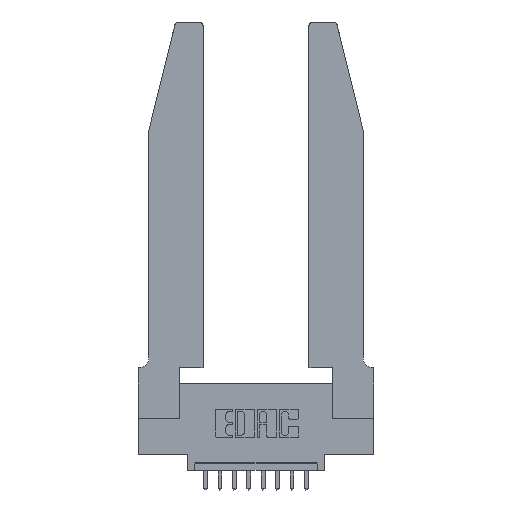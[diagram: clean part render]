
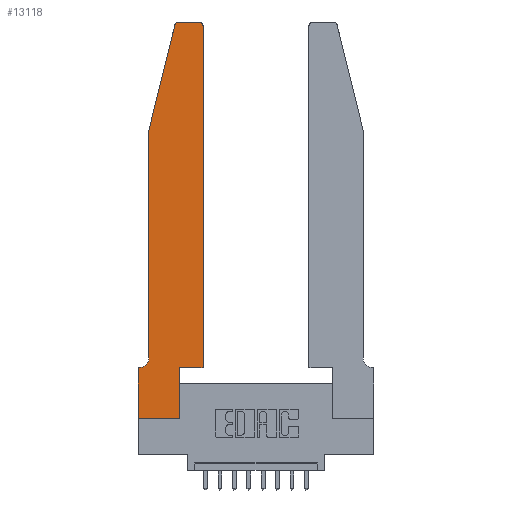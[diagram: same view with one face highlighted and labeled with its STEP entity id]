
A CAD part, top view. The second image highlights one B-rep face of the part: STEP entity #13118.
In plain terms, the highlighted planar face has unit normal (0, 0, 1).
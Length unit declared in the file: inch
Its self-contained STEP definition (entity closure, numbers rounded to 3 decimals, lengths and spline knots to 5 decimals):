
#37 = CARTESIAN_POINT ( 'NONE',  ( 0.0055, 0.42, 0.37 ) ) ;
#318 = ORIENTED_EDGE ( 'NONE', *, *, #5589, .T. ) ;
#415 = VECTOR ( 'NONE', #8741, 39.37008 ) ;
#494 = ORIENTED_EDGE ( 'NONE', *, *, #6940, .T. ) ;
#845 = ORIENTED_EDGE ( 'NONE', *, *, #9749, .T. ) ;
#1042 = DIRECTION ( 'NONE',  ( 0., 0., 1. ) ) ;
#1146 = CARTESIAN_POINT ( 'NONE',  ( 0.284, 2.72, 0.37 ) ) ;
#1569 = PLANE ( 'NONE',  #14607 ) ;
#1967 = VERTEX_POINT ( 'NONE', #10057 ) ;
#1981 = CIRCLE ( 'NONE', #5795, 0.07 ) ;
#2119 = VERTEX_POINT ( 'NONE', #8149 ) ;
#2157 = EDGE_CURVE ( 'NONE', #10383, #11091, #13105, .T. ) ;
#2395 = ORIENTED_EDGE ( 'NONE', *, *, #12635, .T. ) ;
#2625 = VECTOR ( 'NONE', #10689, 39.37008 ) ;
#2640 = VERTEX_POINT ( 'NONE', #8347 ) ;
#2747 = VERTEX_POINT ( 'NONE', #4950 ) ;
#2975 = FACE_OUTER_BOUND ( 'NONE', #6156, .T. ) ;
#3024 = CARTESIAN_POINT ( 'NONE',  ( 0.4505, 2.72, 0.37 ) ) ;
#3044 = AXIS2_PLACEMENT_3D ( 'NONE', #1146, #1042, #4704 ) ;
#3399 = EDGE_CURVE ( 'NONE', #11091, #9227, #14412, .T. ) ;
#3501 = DIRECTION ( 'NONE',  ( -0.239, -0.971, 0. ) ) ;
#3554 = VECTOR ( 'NONE', #3501, 39.37008 ) ;
#3577 = LINE ( 'NONE', #6527, #7161 ) ;
#3654 = DIRECTION ( 'NONE',  ( 0., 1., 0. ) ) ;
#3967 = CARTESIAN_POINT ( 'NONE',  ( 0., 0.35, 0.37 ) ) ;
#4281 = EDGE_CURVE ( 'NONE', #1967, #6999, #15196, .T. ) ;
#4324 = VECTOR ( 'NONE', #12810, 39.37008 ) ;
#4589 = ORIENTED_EDGE ( 'NONE', *, *, #2157, .T. ) ;
#4704 = DIRECTION ( 'NONE',  ( 1., 0., 0. ) ) ;
#4751 = DIRECTION ( 'NONE',  ( -1., 0., 0. ) ) ;
#4950 = CARTESIAN_POINT ( 'NONE',  ( 0.0755, 2., 0.37 ) ) ;
#4961 = ORIENTED_EDGE ( 'NONE', *, *, #12602, .T. ) ;
#5038 = CARTESIAN_POINT ( 'NONE',  ( 0.2865, 0.35, 0.37 ) ) ;
#5060 = DIRECTION ( 'NONE',  ( 0., 1., 0. ) ) ;
#5204 = DIRECTION ( 'NONE',  ( 0., 0., 1. ) ) ;
#5482 = CARTESIAN_POINT ( 'NONE',  ( 0.284, 2.75, 0.37 ) ) ;
#5589 = EDGE_CURVE ( 'NONE', #2747, #2640, #9210, .T. ) ;
#5600 = ORIENTED_EDGE ( 'NONE', *, *, #12758, .T. ) ;
#5795 = AXIS2_PLACEMENT_3D ( 'NONE', #37, #8422, #10828 ) ;
#6007 = LINE ( 'NONE', #9488, #2625 ) ;
#6156 = EDGE_LOOP ( 'NONE', ( #14097, #5600, #4961, #318, #7745, #8527, #8144, #2395, #845, #494, #11410, #4589 ) ) ;
#6436 = DIRECTION ( 'NONE',  ( 0., -1., 0. ) ) ;
#6527 = CARTESIAN_POINT ( 'NONE',  ( 0., 0., 0.37 ) ) ;
#6940 = EDGE_CURVE ( 'NONE', #12651, #11143, #6007, .T. ) ;
#6999 = VERTEX_POINT ( 'NONE', #10043 ) ;
#7033 = CARTESIAN_POINT ( 'NONE',  ( 0.25487, 2.72718, 0.37 ) ) ;
#7161 = VECTOR ( 'NONE', #6436, 39.37008 ) ;
#7534 = VECTOR ( 'NONE', #3654, 39.37008 ) ;
#7745 = ORIENTED_EDGE ( 'NONE', *, *, #15525, .T. ) ;
#8099 = CARTESIAN_POINT ( 'NONE',  ( 0.4205, 2.72, 0.37 ) ) ;
#8144 = ORIENTED_EDGE ( 'NONE', *, *, #11043, .T. ) ;
#8149 = CARTESIAN_POINT ( 'NONE',  ( 0.2865, 0., 0.37 ) ) ;
#8242 = AXIS2_PLACEMENT_3D ( 'NONE', #8099, #12911, #14119 ) ;
#8347 = CARTESIAN_POINT ( 'NONE',  ( 0.0755, 0.42, 0.37 ) ) ;
#8422 = DIRECTION ( 'NONE',  ( 0., 0., -1. ) ) ;
#8527 = ORIENTED_EDGE ( 'NONE', *, *, #4281, .T. ) ;
#8741 = DIRECTION ( 'NONE',  ( -1., 0., 0. ) ) ;
#8923 = VERTEX_POINT ( 'NONE', #7033 ) ;
#8940 = CARTESIAN_POINT ( 'NONE',  ( 0.0755, 0.35, 0.37 ) ) ;
#8990 = VECTOR ( 'NONE', #9888, 39.37008 ) ;
#9210 = LINE ( 'NONE', #10341, #4324 ) ;
#9227 = VERTEX_POINT ( 'NONE', #5482 ) ;
#9481 = CARTESIAN_POINT ( 'NONE',  ( 0.0755, 2., 0.37 ) ) ;
#9488 = CARTESIAN_POINT ( 'NONE',  ( 0.4505, 0.35, 0.37 ) ) ;
#9523 = CARTESIAN_POINT ( 'NONE',  ( 0.2605, 2.75, 0.37 ) ) ;
#9749 = EDGE_CURVE ( 'NONE', #2119, #12651, #11343, .T. ) ;
#9888 = DIRECTION ( 'NONE',  ( 1., 0., 0. ) ) ;
#10043 = CARTESIAN_POINT ( 'NONE',  ( 0., 0.35, 0.37 ) ) ;
#10057 = CARTESIAN_POINT ( 'NONE',  ( 0.0055, 0.35, 0.37 ) ) ;
#10307 = LINE ( 'NONE', #9481, #3554 ) ;
#10341 = CARTESIAN_POINT ( 'NONE',  ( 0.0755, 2., 0.37 ) ) ;
#10383 = VERTEX_POINT ( 'NONE', #3024 ) ;
#10608 = CARTESIAN_POINT ( 'NONE',  ( 0.4505, 0.35, 0.37 ) ) ;
#10689 = DIRECTION ( 'NONE',  ( 1., 0., 0. ) ) ;
#10692 = LINE ( 'NONE', #10838, #7534 ) ;
#10828 = DIRECTION ( 'NONE',  ( -1., 0., 0. ) ) ;
#10838 = CARTESIAN_POINT ( 'NONE',  ( 0.4505, 0.35, 0.37 ) ) ;
#10893 = CARTESIAN_POINT ( 'NONE',  ( 0., 0., 0.37 ) ) ;
#11043 = EDGE_CURVE ( 'NONE', #6999, #12601, #3577, .T. ) ;
#11087 = LINE ( 'NONE', #10893, #8990 ) ;
#11091 = VERTEX_POINT ( 'NONE', #13747 ) ;
#11143 = VERTEX_POINT ( 'NONE', #10608 ) ;
#11153 = VECTOR ( 'NONE', #5060, 39.37008 ) ;
#11252 = CIRCLE ( 'NONE', #3044, 0.03 ) ;
#11343 = LINE ( 'NONE', #13457, #11153 ) ;
#11410 = ORIENTED_EDGE ( 'NONE', *, *, #12582, .T. ) ;
#11848 = CARTESIAN_POINT ( 'NONE',  ( 0., 0., 0.37 ) ) ;
#12582 = EDGE_CURVE ( 'NONE', #11143, #10383, #10692, .T. ) ;
#12601 = VERTEX_POINT ( 'NONE', #11848 ) ;
#12602 = EDGE_CURVE ( 'NONE', #8923, #2747, #10307, .T. ) ;
#12635 = EDGE_CURVE ( 'NONE', #12601, #2119, #11087, .T. ) ;
#12651 = VERTEX_POINT ( 'NONE', #5038 ) ;
#12758 = EDGE_CURVE ( 'NONE', #9227, #8923, #11252, .T. ) ;
#12810 = DIRECTION ( 'NONE',  ( 0., -1., 0. ) ) ;
#12911 = DIRECTION ( 'NONE',  ( 0., 0., 1. ) ) ;
#13105 = CIRCLE ( 'NONE', #8242, 0.03 ) ;
#13118 = ADVANCED_FACE ( 'NONE', ( #2975 ), #1569, .T. ) ;
#13457 = CARTESIAN_POINT ( 'NONE',  ( 0.2865, 0.35, 0.37 ) ) ;
#13661 = VECTOR ( 'NONE', #4751, 39.37008 ) ;
#13747 = CARTESIAN_POINT ( 'NONE',  ( 0.4205, 2.75, 0.37 ) ) ;
#14097 = ORIENTED_EDGE ( 'NONE', *, *, #3399, .T. ) ;
#14119 = DIRECTION ( 'NONE',  ( 1., 0., 0. ) ) ;
#14412 = LINE ( 'NONE', #9523, #13661 ) ;
#14607 = AXIS2_PLACEMENT_3D ( 'NONE', #3967, #5204, #14777 ) ;
#14777 = DIRECTION ( 'NONE',  ( 1., 0., 0. ) ) ;
#15196 = LINE ( 'NONE', #8940, #415 ) ;
#15525 = EDGE_CURVE ( 'NONE', #2640, #1967, #1981, .T. ) ;
